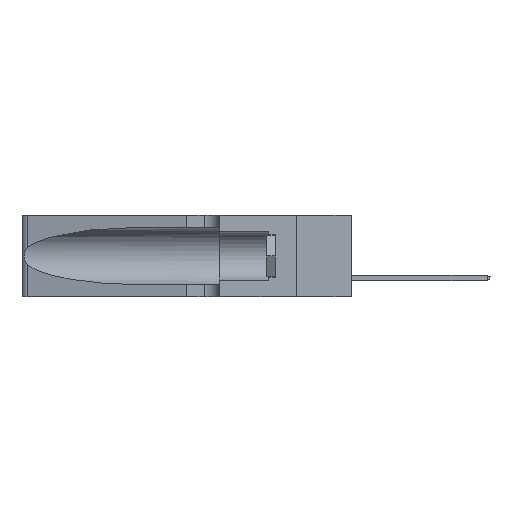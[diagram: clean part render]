
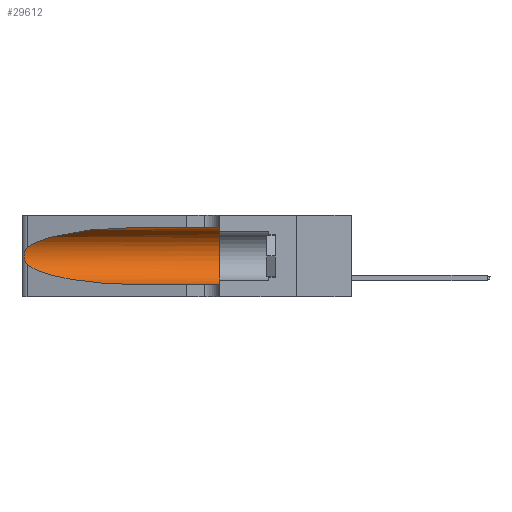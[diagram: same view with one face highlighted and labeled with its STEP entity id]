
A CAD part, left-side view. The second image highlights one B-rep face of the part: STEP entity #29612.
In plain terms, the highlighted cylindrical face has radius 3.308 mm (diameter 6.617 mm), a partial arc.
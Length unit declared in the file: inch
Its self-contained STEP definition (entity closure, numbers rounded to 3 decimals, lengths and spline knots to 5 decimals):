
#303 = VERTEX_POINT ( 'NONE', #9196 ) ;
#601 = CARTESIAN_POINT ( 'NONE',  ( 0.26017, 1.23833, 0.17102 ) ) ;
#1957 = VERTEX_POINT ( 'NONE', #4769 ) ;
#2332 = CARTESIAN_POINT ( 'NONE',  ( 0.2373, 1.15595, 0.28018 ) ) ;
#2344 = CARTESIAN_POINT ( 'NONE',  ( 0.2373, 1.15595, 0.08982 ) ) ;
#4283 = CARTESIAN_POINT ( 'NONE',  ( 0.25856, 1.23593, 0.16098 ) ) ;
#4769 = CARTESIAN_POINT ( 'NONE',  ( 0.1305, 0.72297, 0.31525 ) ) ;
#5486 = ORIENTED_EDGE ( 'NONE', *, *, #12880, .T. ) ;
#5562 = CARTESIAN_POINT ( 'NONE',  ( 0.18966, 0.96281, 0.05475 ) ) ;
#5905 = CARTESIAN_POINT ( 'NONE',  ( 0.1305, 0.35, 0.05475 ) ) ;
#6184 = FACE_OUTER_BOUND ( 'NONE', #35470, .T. ) ;
#6628 = EDGE_CURVE ( 'NONE', #14266, #39150, #42170, .T. ) ;
#6983 =( BOUNDED_CURVE ( )  B_SPLINE_CURVE ( 3, ( #13388, #2344, #5562, #24451 ),
 .UNSPECIFIED., .F., .T. ) 
 B_SPLINE_CURVE_WITH_KNOTS ( ( 4, 4 ),
 ( 3.44316, 4.71239 ),
 .UNSPECIFIED. ) 
 CURVE ( )  GEOMETRIC_REPRESENTATION_ITEM ( )  RATIONAL_B_SPLINE_CURVE ( ( 1., 0.87, 0.87, 1. ) ) 
 REPRESENTATION_ITEM ( '' )  );
#8512 = AXIS2_PLACEMENT_3D ( 'NONE', #40748, #11636, #38483 ) ;
#8790 = B_SPLINE_CURVE_WITH_KNOTS ( 'NONE', 3,
 ( #11141, #33380, #11764, #40729, #29393, #22561, #18539, #15311, #601, #4283, #40877, #37355, #44068, #16109 ),
 .UNSPECIFIED., .F., .F.,
 ( 4, 2, 2, 2, 2, 2, 4 ),
 ( 0., 0.00027, 0.00053, 0.00107, 0.0016, 0.00187, 0.00214 ),
 .UNSPECIFIED. ) ;
#9196 = CARTESIAN_POINT ( 'NONE',  ( 0.25487, 1.22718, 0.22369 ) ) ;
#11141 = CARTESIAN_POINT ( 'NONE',  ( 0.25487, 1.22718, 0.22369 ) ) ;
#11636 = DIRECTION ( 'NONE',  ( 0., 1., 0. ) ) ;
#11764 = CARTESIAN_POINT ( 'NONE',  ( 0.25639, 1.23184, 0.21858 ) ) ;
#12880 = EDGE_CURVE ( 'NONE', #47210, #39150, #43695, .T. ) ;
#13388 = CARTESIAN_POINT ( 'NONE',  ( 0.25487, 1.22718, 0.14631 ) ) ;
#13563 = ORIENTED_EDGE ( 'NONE', *, *, #19491, .F. ) ;
#14266 = VERTEX_POINT ( 'NONE', #21671 ) ;
#14602 = VECTOR ( 'NONE', #37845, 39.37008 ) ;
#15311 = CARTESIAN_POINT ( 'NONE',  ( 0.26075, 1.23896, 0.178 ) ) ;
#15654 = EDGE_CURVE ( 'NONE', #303, #19317, #8790, .T. ) ;
#16109 = CARTESIAN_POINT ( 'NONE',  ( 0.25487, 1.22718, 0.14631 ) ) ;
#16918 = CARTESIAN_POINT ( 'NONE',  ( 0.1305, 0.72297, 0.31525 ) ) ;
#18476 = DIRECTION ( 'NONE',  ( 0., -1., 0. ) ) ;
#18539 = CARTESIAN_POINT ( 'NONE',  ( 0.26075, 1.23896, 0.19203 ) ) ;
#18806 = AXIS2_PLACEMENT_3D ( 'NONE', #40813, #18476, #36995 ) ;
#19158 = CARTESIAN_POINT ( 'NONE',  ( 0.1305, 1.61858, 0.31525 ) ) ;
#19317 = VERTEX_POINT ( 'NONE', #31641 ) ;
#19491 = EDGE_CURVE ( 'NONE', #1957, #14266, #36353, .T. ) ;
#20301 = CARTESIAN_POINT ( 'NONE',  ( 0.25487, 1.22718, 0.22369 ) ) ;
#21671 = CARTESIAN_POINT ( 'NONE',  ( 0.1305, 0.35, 0.31525 ) ) ;
#22561 = CARTESIAN_POINT ( 'NONE',  ( 0.26018, 1.23835, 0.19895 ) ) ;
#22833 = ORIENTED_EDGE ( 'NONE', *, *, #46110, .T. ) ;
#24451 = CARTESIAN_POINT ( 'NONE',  ( 0.1305, 0.72297, 0.05475 ) ) ;
#24985 = ORIENTED_EDGE ( 'NONE', *, *, #6628, .F. ) ;
#27626 = CARTESIAN_POINT ( 'NONE',  ( 0.1305, 0.72297, 0.05475 ) ) ;
#29393 = CARTESIAN_POINT ( 'NONE',  ( 0.25854, 1.2359, 0.20912 ) ) ;
#29612 = ADVANCED_FACE ( 'NONE', ( #6184 ), #33106, .F. ) ;
#31317 = CARTESIAN_POINT ( 'NONE',  ( 0.18966, 0.96281, 0.31525 ) ) ;
#31641 = CARTESIAN_POINT ( 'NONE',  ( 0.25487, 1.22718, 0.14631 ) ) ;
#33106 = CYLINDRICAL_SURFACE ( 'NONE', #18806, 0.13025 ) ;
#33380 = CARTESIAN_POINT ( 'NONE',  ( 0.25555, 1.22994, 0.2215 ) ) ;
#34467 = CARTESIAN_POINT ( 'NONE',  ( 0.1305, 1.61858, 0.05475 ) ) ;
#35470 = EDGE_LOOP ( 'NONE', ( #22833, #45429, #37467, #5486, #24985, #13563 ) ) ;
#36353 = LINE ( 'NONE', #19158, #14602 ) ;
#36995 = DIRECTION ( 'NONE',  ( 0., 0., -1. ) ) ;
#37355 = CARTESIAN_POINT ( 'NONE',  ( 0.25639, 1.23186, 0.15144 ) ) ;
#37417 = VECTOR ( 'NONE', #38638, 39.37008 ) ;
#37467 = ORIENTED_EDGE ( 'NONE', *, *, #47167, .T. ) ;
#37845 = DIRECTION ( 'NONE',  ( 0., -1., 0. ) ) ;
#38483 = DIRECTION ( 'NONE',  ( 0., 0., 1. ) ) ;
#38638 = DIRECTION ( 'NONE',  ( 0., -1., 0. ) ) ;
#39150 = VERTEX_POINT ( 'NONE', #5905 ) ;
#40134 =( BOUNDED_CURVE ( )  B_SPLINE_CURVE ( 3, ( #16918, #31317, #2332, #20301 ),
 .UNSPECIFIED., .F., .T. ) 
 B_SPLINE_CURVE_WITH_KNOTS ( ( 4, 4 ),
 ( 1.5708, 2.84003 ),
 .UNSPECIFIED. ) 
 CURVE ( )  GEOMETRIC_REPRESENTATION_ITEM ( )  RATIONAL_B_SPLINE_CURVE ( ( 1., 0.87, 0.87, 1. ) ) 
 REPRESENTATION_ITEM ( '' )  );
#40729 = CARTESIAN_POINT ( 'NONE',  ( 0.25787, 1.23484, 0.2124 ) ) ;
#40748 = CARTESIAN_POINT ( 'NONE',  ( 0.1305, 0.35, 0.185 ) ) ;
#40813 = CARTESIAN_POINT ( 'NONE',  ( 0.1305, 1.61858, 0.185 ) ) ;
#40877 = CARTESIAN_POINT ( 'NONE',  ( 0.25789, 1.23486, 0.15765 ) ) ;
#42170 = CIRCLE ( 'NONE', #8512, 0.13025 ) ;
#43695 = LINE ( 'NONE', #34467, #37417 ) ;
#44068 = CARTESIAN_POINT ( 'NONE',  ( 0.25555, 1.22993, 0.14849 ) ) ;
#45429 = ORIENTED_EDGE ( 'NONE', *, *, #15654, .T. ) ;
#46110 = EDGE_CURVE ( 'NONE', #1957, #303, #40134, .T. ) ;
#47167 = EDGE_CURVE ( 'NONE', #19317, #47210, #6983, .T. ) ;
#47210 = VERTEX_POINT ( 'NONE', #27626 ) ;
